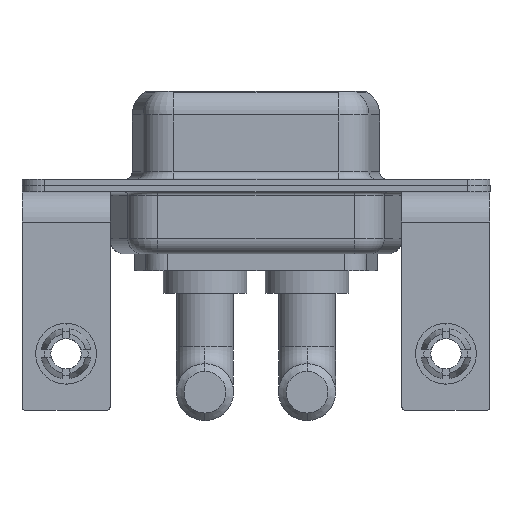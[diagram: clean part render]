
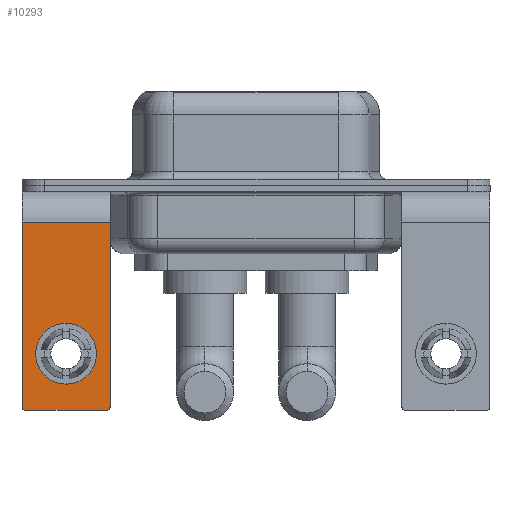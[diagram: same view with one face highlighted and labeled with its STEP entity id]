
A CAD part, front view. The second image highlights one B-rep face of the part: STEP entity #10293.
In plain terms, the highlighted planar face has unit normal (0, -1, 0).
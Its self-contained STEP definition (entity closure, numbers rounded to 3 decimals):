
#37 = CARTESIAN_POINT ( 'NONE',  ( 2.9, -6.25, -2.4 ) ) ;
#109 = DIRECTION ( 'NONE',  ( 0., 0., -1. ) ) ;
#211 = ORIENTED_EDGE ( 'NONE', *, *, #11220, .T. ) ;
#311 = DIRECTION ( 'NONE',  ( 0., 1., 0. ) ) ;
#331 = CARTESIAN_POINT ( 'NONE',  ( 2.9, -6.25, -14.55 ) ) ;
#551 = EDGE_CURVE ( 'NONE', #12442, #12745, #6881, .T. ) ;
#578 = LINE ( 'NONE', #5308, #13460 ) ;
#1108 = CARTESIAN_POINT ( 'NONE',  ( -2.9, -6.25, -2.4 ) ) ;
#1109 = VERTEX_POINT ( 'NONE', #10503 ) ;
#1336 = CARTESIAN_POINT ( 'NONE',  ( 2.9, -6.25, -2.4 ) ) ;
#1492 = DIRECTION ( 'NONE',  ( 0., 0., 1. ) ) ;
#1505 = DIRECTION ( 'NONE',  ( 0., 0., 1. ) ) ;
#1781 = ORIENTED_EDGE ( 'NONE', *, *, #10488, .T. ) ;
#1924 = AXIS2_PLACEMENT_3D ( 'NONE', #11082, #3899, #9426 ) ;
#2672 = EDGE_CURVE ( 'NONE', #7719, #7938, #6985, .T. ) ;
#3204 = VERTEX_POINT ( 'NONE', #12534 ) ;
#3542 = ORIENTED_EDGE ( 'NONE', *, *, #3940, .F. ) ;
#3549 = DIRECTION ( 'NONE',  ( 0., 0., -1. ) ) ;
#3899 = DIRECTION ( 'NONE',  ( 0., 1., 0. ) ) ;
#3940 = EDGE_CURVE ( 'NONE', #12442, #7938, #5652, .T. ) ;
#3942 = VECTOR ( 'NONE', #109, 1000. ) ;
#3975 = CARTESIAN_POINT ( 'NONE',  ( -2.65, -6.25, -14.8 ) ) ;
#4585 = EDGE_CURVE ( 'NONE', #12745, #13647, #13786, .T. ) ;
#4601 = CARTESIAN_POINT ( 'NONE',  ( -2.9, -6.25, -2.4 ) ) ;
#4918 = CIRCLE ( 'NONE', #8912, 2. ) ;
#5240 = AXIS2_PLACEMENT_3D ( 'NONE', #13876, #8210, #1505 ) ;
#5308 = CARTESIAN_POINT ( 'NONE',  ( 2.9, -6.25, -14.8 ) ) ;
#5647 = VERTEX_POINT ( 'NONE', #3975 ) ;
#5652 = LINE ( 'NONE', #37, #3942 ) ;
#5833 = AXIS2_PLACEMENT_3D ( 'NONE', #9803, #13183, #8476 ) ;
#6038 = AXIS2_PLACEMENT_3D ( 'NONE', #7739, #12515, #6565 ) ;
#6115 = EDGE_LOOP ( 'NONE', ( #7785, #211, #10106, #6824, #3542, #12839 ) ) ;
#6188 = PLANE ( 'NONE',  #1924 ) ;
#6189 = DIRECTION ( 'NONE',  ( -1., 0., 0. ) ) ;
#6565 = DIRECTION ( 'NONE',  ( 0., 0., 1. ) ) ;
#6608 = FACE_BOUND ( 'NONE', #7531, .T. ) ;
#6824 = ORIENTED_EDGE ( 'NONE', *, *, #2672, .T. ) ;
#6881 = LINE ( 'NONE', #1336, #14193 ) ;
#6985 = CIRCLE ( 'NONE', #6038, 0.25 ) ;
#7064 = EDGE_CURVE ( 'NONE', #1109, #3204, #4918, .T. ) ;
#7467 = CIRCLE ( 'NONE', #5833, 0.25 ) ;
#7531 = EDGE_LOOP ( 'NONE', ( #10793, #1781 ) ) ;
#7719 = VERTEX_POINT ( 'NONE', #10946 ) ;
#7725 = VECTOR ( 'NONE', #3549, 1000. ) ;
#7739 = CARTESIAN_POINT ( 'NONE',  ( 2.65, -6.25, -14.55 ) ) ;
#7785 = ORIENTED_EDGE ( 'NONE', *, *, #4585, .T. ) ;
#7938 = VERTEX_POINT ( 'NONE', #331 ) ;
#8210 = DIRECTION ( 'NONE',  ( 0., 1., 0. ) ) ;
#8457 = FACE_OUTER_BOUND ( 'NONE', #6115, .T. ) ;
#8476 = DIRECTION ( 'NONE',  ( 0., 0., 1. ) ) ;
#8912 = AXIS2_PLACEMENT_3D ( 'NONE', #11658, #311, #1492 ) ;
#9426 = DIRECTION ( 'NONE',  ( 0., 0., 1. ) ) ;
#9803 = CARTESIAN_POINT ( 'NONE',  ( -2.65, -6.25, -14.55 ) ) ;
#10106 = ORIENTED_EDGE ( 'NONE', *, *, #11654, .F. ) ;
#10293 = ADVANCED_FACE ( 'NONE', ( #6608, #8457 ), #6188, .F. ) ;
#10488 = EDGE_CURVE ( 'NONE', #3204, #1109, #10630, .T. ) ;
#10503 = CARTESIAN_POINT ( 'NONE',  ( 0., -6.25, -13.07 ) ) ;
#10630 = CIRCLE ( 'NONE', #5240, 2. ) ;
#10793 = ORIENTED_EDGE ( 'NONE', *, *, #7064, .T. ) ;
#10946 = CARTESIAN_POINT ( 'NONE',  ( 2.65, -6.25, -14.8 ) ) ;
#11082 = CARTESIAN_POINT ( 'NONE',  ( 2.9, -6.25, -2.4 ) ) ;
#11220 = EDGE_CURVE ( 'NONE', #13647, #5647, #7467, .T. ) ;
#11574 = DIRECTION ( 'NONE',  ( -1., 0., 0. ) ) ;
#11654 = EDGE_CURVE ( 'NONE', #7719, #5647, #578, .T. ) ;
#11658 = CARTESIAN_POINT ( 'NONE',  ( 0., -6.25, -11.07 ) ) ;
#12348 = CARTESIAN_POINT ( 'NONE',  ( -2.9, -6.25, -14.55 ) ) ;
#12442 = VERTEX_POINT ( 'NONE', #13930 ) ;
#12515 = DIRECTION ( 'NONE',  ( 0., -1., 0. ) ) ;
#12534 = CARTESIAN_POINT ( 'NONE',  ( 0., -6.25, -9.07 ) ) ;
#12745 = VERTEX_POINT ( 'NONE', #1108 ) ;
#12839 = ORIENTED_EDGE ( 'NONE', *, *, #551, .T. ) ;
#13183 = DIRECTION ( 'NONE',  ( 0., -1., 0. ) ) ;
#13460 = VECTOR ( 'NONE', #6189, 1000. ) ;
#13647 = VERTEX_POINT ( 'NONE', #12348 ) ;
#13786 = LINE ( 'NONE', #4601, #7725 ) ;
#13876 = CARTESIAN_POINT ( 'NONE',  ( 0., -6.25, -11.07 ) ) ;
#13930 = CARTESIAN_POINT ( 'NONE',  ( 2.9, -6.25, -2.4 ) ) ;
#14193 = VECTOR ( 'NONE', #11574, 1000. ) ;
